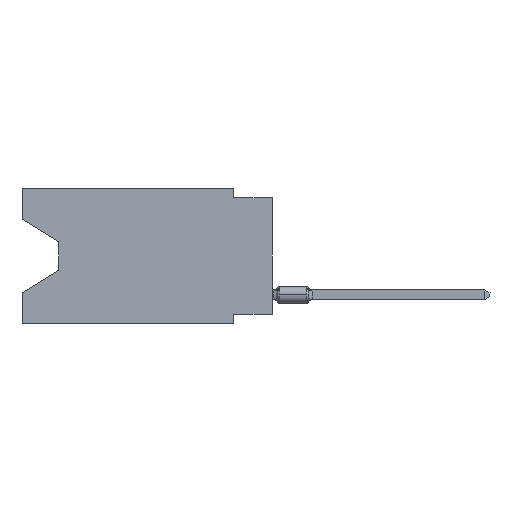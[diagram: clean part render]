
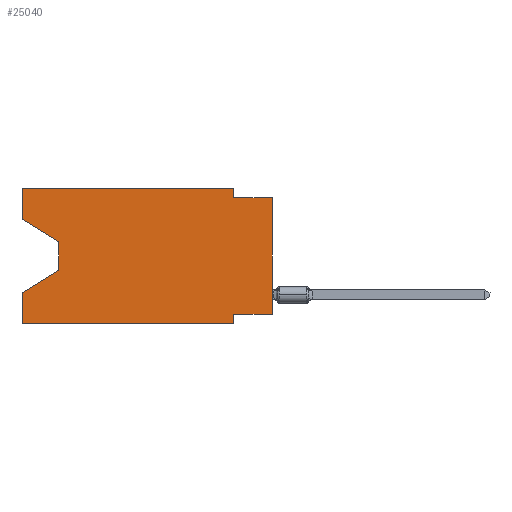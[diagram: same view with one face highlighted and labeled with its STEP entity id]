
A CAD part, left-side view. The second image highlights one B-rep face of the part: STEP entity #25040.
In plain terms, the highlighted planar face has unit normal (-1, 0, 0).
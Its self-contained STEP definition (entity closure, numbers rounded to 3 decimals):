
#193 = CARTESIAN_POINT ( 'NONE',  ( 0., 16.383, 0. ) ) ;
#243 = ORIENTED_EDGE ( 'NONE', *, *, #27567, .T. ) ;
#384 = CARTESIAN_POINT ( 'NONE',  ( 0., 13.97, -5.385 ) ) ;
#442 = ORIENTED_EDGE ( 'NONE', *, *, #16356, .F. ) ;
#660 = CARTESIAN_POINT ( 'NONE',  ( 0., 16.383, -6.852 ) ) ;
#777 = VECTOR ( 'NONE', #8732, 1000. ) ;
#1395 = CARTESIAN_POINT ( 'NONE',  ( 0., 2.54, -8.89 ) ) ;
#1480 = LINE ( 'NONE', #24702, #2208 ) ;
#1849 = ORIENTED_EDGE ( 'NONE', *, *, #25661, .F. ) ;
#1912 = CARTESIAN_POINT ( 'NONE',  ( 0., 2.54, -8.255 ) ) ;
#2051 = VERTEX_POINT ( 'NONE', #7865 ) ;
#2208 = VECTOR ( 'NONE', #21861, 1000. ) ;
#2576 = CARTESIAN_POINT ( 'NONE',  ( 0., 16.383, -8.89 ) ) ;
#2897 = PLANE ( 'NONE',  #6864 ) ;
#3137 = EDGE_CURVE ( 'NONE', #22217, #17258, #8944, .T. ) ;
#3588 = CARTESIAN_POINT ( 'NONE',  ( 0., 16.383, -8.89 ) ) ;
#4517 = DIRECTION ( 'NONE',  ( 0., 0., -1. ) ) ;
#4766 = ORIENTED_EDGE ( 'NONE', *, *, #23824, .T. ) ;
#4822 = VECTOR ( 'NONE', #7716, 1000. ) ;
#5060 = LINE ( 'NONE', #384, #19358 ) ;
#5199 = ORIENTED_EDGE ( 'NONE', *, *, #24827, .T. ) ;
#5396 = CARTESIAN_POINT ( 'NONE',  ( 0., 2.54, 0. ) ) ;
#5404 = DIRECTION ( 'NONE',  ( 0., 0., -1. ) ) ;
#5853 = VERTEX_POINT ( 'NONE', #26588 ) ;
#6470 = VECTOR ( 'NONE', #16404, 1000. ) ;
#6864 = AXIS2_PLACEMENT_3D ( 'NONE', #15100, #13088, #5404 ) ;
#6882 = VERTEX_POINT ( 'NONE', #17308 ) ;
#7032 = VECTOR ( 'NONE', #30100, 1000. ) ;
#7044 = VECTOR ( 'NONE', #18803, 1000. ) ;
#7494 = CARTESIAN_POINT ( 'NONE',  ( 0., 0., -0.635 ) ) ;
#7593 = EDGE_LOOP ( 'NONE', ( #17606, #5199, #243, #1849, #15570, #21278, #14828, #4766, #25699, #442, #24896, #25756 ) ) ;
#7716 = DIRECTION ( 'NONE',  ( 0., 0., 1. ) ) ;
#7865 = CARTESIAN_POINT ( 'NONE',  ( 0., 16.383, -2.038 ) ) ;
#8275 = DIRECTION ( 'NONE',  ( 0., 0., -1. ) ) ;
#8732 = DIRECTION ( 'NONE',  ( 0., 1., 0. ) ) ;
#8944 = LINE ( 'NONE', #3588, #31138 ) ;
#9491 = CARTESIAN_POINT ( 'NONE',  ( 0., 0., -8.255 ) ) ;
#10169 = VECTOR ( 'NONE', #13550, 1000. ) ;
#10571 = DIRECTION ( 'NONE',  ( 0., 0.855, -0.519 ) ) ;
#10889 = VERTEX_POINT ( 'NONE', #14272 ) ;
#12129 = VERTEX_POINT ( 'NONE', #28445 ) ;
#13088 = DIRECTION ( 'NONE',  ( 1., 0., 0. ) ) ;
#13228 = CARTESIAN_POINT ( 'NONE',  ( 0., 16.383, -2.038 ) ) ;
#13486 = VERTEX_POINT ( 'NONE', #660 ) ;
#13550 = DIRECTION ( 'NONE',  ( 0., 0., 1. ) ) ;
#13612 = LINE ( 'NONE', #1395, #7044 ) ;
#14272 = CARTESIAN_POINT ( 'NONE',  ( 0., 16.383, 0. ) ) ;
#14828 = ORIENTED_EDGE ( 'NONE', *, *, #31869, .F. ) ;
#15100 = CARTESIAN_POINT ( 'NONE',  ( 0., 16.383, 0. ) ) ;
#15570 = ORIENTED_EDGE ( 'NONE', *, *, #3137, .T. ) ;
#15871 = CARTESIAN_POINT ( 'NONE',  ( 0., 2.54, -8.89 ) ) ;
#16356 = EDGE_CURVE ( 'NONE', #28627, #5853, #29908, .T. ) ;
#16404 = DIRECTION ( 'NONE',  ( 0., -0.855, -0.519 ) ) ;
#16460 = LINE ( 'NONE', #31671, #21263 ) ;
#16795 = EDGE_CURVE ( 'NONE', #5853, #24242, #1480, .T. ) ;
#16918 = EDGE_CURVE ( 'NONE', #2051, #12129, #18918, .T. ) ;
#17258 = VERTEX_POINT ( 'NONE', #15871 ) ;
#17308 = CARTESIAN_POINT ( 'NONE',  ( 0., 13.97, -5.385 ) ) ;
#17606 = ORIENTED_EDGE ( 'NONE', *, *, #16918, .T. ) ;
#18188 = EDGE_CURVE ( 'NONE', #24967, #17258, #13612, .T. ) ;
#18803 = DIRECTION ( 'NONE',  ( 0., 0., -1. ) ) ;
#18918 = LINE ( 'NONE', #13228, #6470 ) ;
#19358 = VECTOR ( 'NONE', #10571, 1000. ) ;
#20384 = VECTOR ( 'NONE', #4517, 1000. ) ;
#20985 = LINE ( 'NONE', #23960, #22833 ) ;
#21060 = EDGE_CURVE ( 'NONE', #2051, #10889, #23070, .T. ) ;
#21263 = VECTOR ( 'NONE', #26323, 1000. ) ;
#21278 = ORIENTED_EDGE ( 'NONE', *, *, #18188, .F. ) ;
#21861 = DIRECTION ( 'NONE',  ( 0., -1., 0. ) ) ;
#22217 = VERTEX_POINT ( 'NONE', #2576 ) ;
#22579 = LINE ( 'NONE', #22728, #7032 ) ;
#22728 = CARTESIAN_POINT ( 'NONE',  ( 0., 0., 0. ) ) ;
#22764 = FACE_OUTER_BOUND ( 'NONE', #7593, .T. ) ;
#22833 = VECTOR ( 'NONE', #8275, 1000. ) ;
#23070 = LINE ( 'NONE', #193, #4822 ) ;
#23386 = CARTESIAN_POINT ( 'NONE',  ( 0., 16.383, 0. ) ) ;
#23824 = EDGE_CURVE ( 'NONE', #30347, #24242, #22579, .T. ) ;
#23960 = CARTESIAN_POINT ( 'NONE',  ( 0., 13.97, -3.505 ) ) ;
#23968 = DIRECTION ( 'NONE',  ( 0., -1., 0. ) ) ;
#24242 = VERTEX_POINT ( 'NONE', #7494 ) ;
#24702 = CARTESIAN_POINT ( 'NONE',  ( 0., 0., -0.635 ) ) ;
#24827 = EDGE_CURVE ( 'NONE', #12129, #6882, #20985, .T. ) ;
#24843 = EDGE_CURVE ( 'NONE', #10889, #28627, #16460, .T. ) ;
#24896 = ORIENTED_EDGE ( 'NONE', *, *, #24843, .F. ) ;
#24967 = VERTEX_POINT ( 'NONE', #1912 ) ;
#25040 = ADVANCED_FACE ( 'NONE', ( #22764 ), #2897, .F. ) ;
#25661 = EDGE_CURVE ( 'NONE', #22217, #13486, #31258, .T. ) ;
#25699 = ORIENTED_EDGE ( 'NONE', *, *, #16795, .F. ) ;
#25756 = ORIENTED_EDGE ( 'NONE', *, *, #21060, .F. ) ;
#26323 = DIRECTION ( 'NONE',  ( 0., -1., 0. ) ) ;
#26516 = CARTESIAN_POINT ( 'NONE',  ( 0., 0., -8.255 ) ) ;
#26588 = CARTESIAN_POINT ( 'NONE',  ( 0., 2.54, -0.635 ) ) ;
#27406 = CARTESIAN_POINT ( 'NONE',  ( 0., 2.54, 0. ) ) ;
#27567 = EDGE_CURVE ( 'NONE', #6882, #13486, #5060, .T. ) ;
#28445 = CARTESIAN_POINT ( 'NONE',  ( 0., 13.97, -3.505 ) ) ;
#28627 = VERTEX_POINT ( 'NONE', #5396 ) ;
#29110 = LINE ( 'NONE', #9491, #777 ) ;
#29908 = LINE ( 'NONE', #27406, #20384 ) ;
#30100 = DIRECTION ( 'NONE',  ( 0., 0., 1. ) ) ;
#30347 = VERTEX_POINT ( 'NONE', #26516 ) ;
#31138 = VECTOR ( 'NONE', #23968, 1000. ) ;
#31258 = LINE ( 'NONE', #23386, #10169 ) ;
#31671 = CARTESIAN_POINT ( 'NONE',  ( 0., 16.383, 0. ) ) ;
#31869 = EDGE_CURVE ( 'NONE', #30347, #24967, #29110, .T. ) ;
